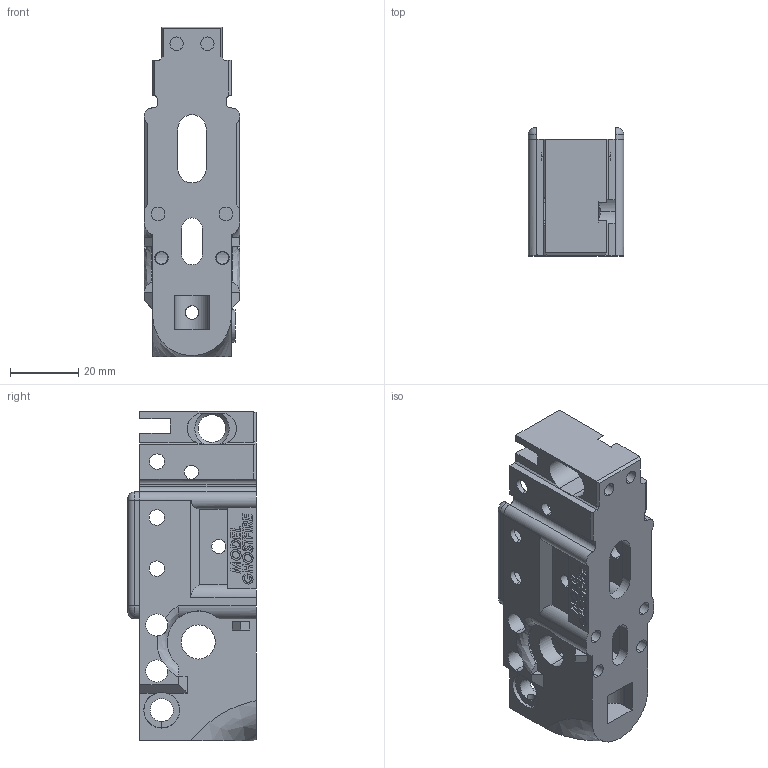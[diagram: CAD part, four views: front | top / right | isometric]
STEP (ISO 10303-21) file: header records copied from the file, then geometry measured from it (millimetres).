
FILE_DESCRIPTION (( 'STEP AP203' ), '1' );
FILE_NAME ('FireControlGroup.STEP', '2019-09-03T07:05:54', ( '' ), ( '' ), 'SwSTEP 2.0', 'SolidWorks 2018', '' );
FILE_SCHEMA (( 'CONFIG_CONTROL_DESIGN' ));
Products named in the file (1): FireControlGroup
Bounding box: 28.07 x 37.65 x 96.7 mm (x, y, z)
Volume: 34139.4 mm3; surface area: 23870.6 mm2
Topology: 1 solids, 32 shells, 1327 faces, 3591 edges, 2387 vertices
Faces by surface type: plane 805, bspline 376, cylinder 140, torus 4, cone 2
Entity records: 60421 total; most frequent: CARTESIAN_POINT 29198, ORIENTED_EDGE 7182, DIRECTION 4986, EDGE_CURVE 3591, VECTOR 2466, LINE 2466, VERTEX_POINT 2387, EDGE_LOOP 1490
